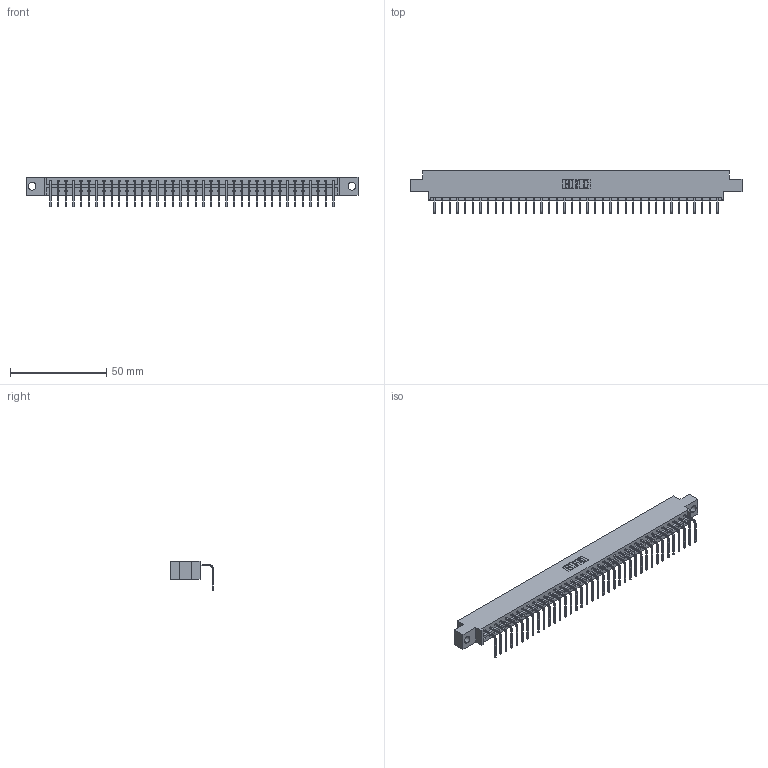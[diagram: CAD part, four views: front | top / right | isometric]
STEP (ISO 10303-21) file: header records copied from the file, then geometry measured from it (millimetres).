
FILE_DESCRIPTION (( 'STEP AP203' ), '1' );
FILE_NAME ('333-038-558-604.STEP', '2018-08-03T12:05:26', ( '' ), ( '' ), 'SwSTEP 2.0', 'SolidWorks 2016', '' );
FILE_SCHEMA (( 'CONFIG_CONTROL_DESIGN' ));
Length unit declared in the file: inch
Products named in the file (3): 333 Part_Offset - .156 Dia - TH; 345-292-001_558 Tail - 2; 333-038-558-604
Assembly tree (39 placements, depth 2):
  333-038-558-604
    333 Part_Offset - .156 Dia - TH
    345-292-001_558 Tail - 2  x38
Bounding box: 172.11 x 22.17 x 15.37 mm (x, y, z)
Volume: 17095.7 mm3; surface area: 19240.8 mm2
Topology: 39 solids, 39 shells, 2398 faces, 7239 edges, 4774 vertices
Faces by surface type: plane 1746, cylinder 652
Entity records: 23967 total; most frequent: CARTESIAN_POINT 4144, ORIENTED_EDGE 4118, DIRECTION 3503, EDGE_CURVE 2059, VECTOR 1931, LINE 1931, VERTEX_POINT 1370, AXIS2_PLACEMENT_3D 786
